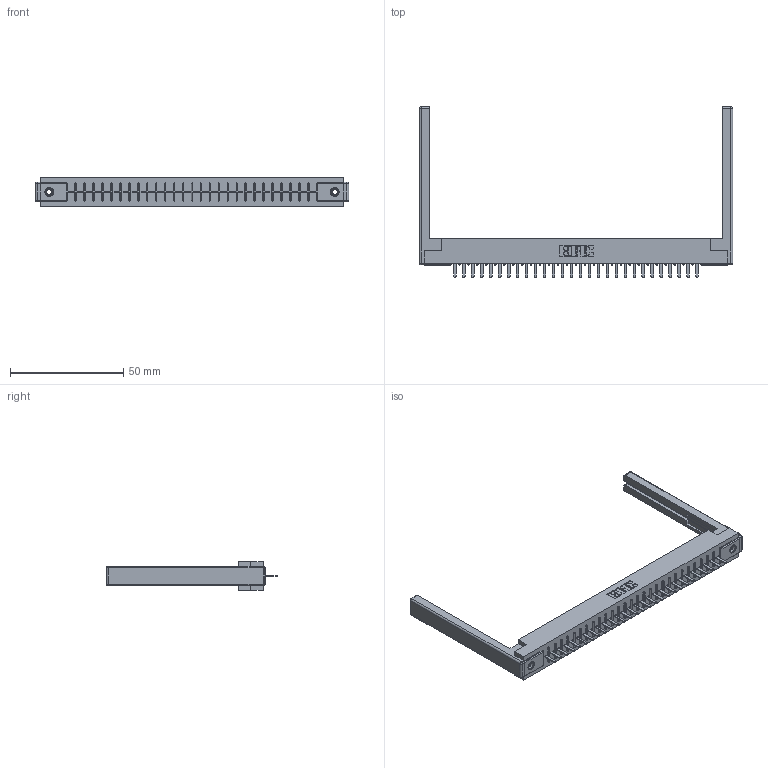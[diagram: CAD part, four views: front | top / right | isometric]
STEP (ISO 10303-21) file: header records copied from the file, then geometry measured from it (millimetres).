
FILE_DESCRIPTION (( 'STEP AP203' ), '1' );
FILE_NAME ('316-028-420-168.STEP', '2020-09-22T23:33:03', ( '' ), ( '' ), 'SwSTEP 2.0', 'SolidWorks 2020', '' );
FILE_SCHEMA (( 'CONFIG_CONTROL_DESIGN' ));
Length unit declared in the file: inch
Products named in the file (5): 306 Part_.156 Dia; 345-250-001_345-250-001-102; 316-028-420-168; 307-220-068; 306-290-001_120
Assembly tree (33 placements, depth 2):
  316-028-420-168
    306 Part_.156 Dia
    306-290-001_120  x28
    345-250-001_345-250-001-102  x2
    307-220-068  x2
Bounding box: 138.38 x 75.41 x 12.7 mm (x, y, z)
Volume: 19545.9 mm3; surface area: 19494.4 mm2
Topology: 33 solids, 33 shells, 2230 faces, 6222 edges, 3976 vertices
Faces by surface type: plane 1472, cylinder 622, sphere 120, cone 12, torus 4
Entity records: 30640 total; most frequent: CARTESIAN_POINT 5108, ORIENTED_EDGE 5054, DIRECTION 5051, EDGE_CURVE 2527, VECTOR 1965, LINE 1965, VERTEX_POINT 1600, AXIS2_PLACEMENT_3D 1543
